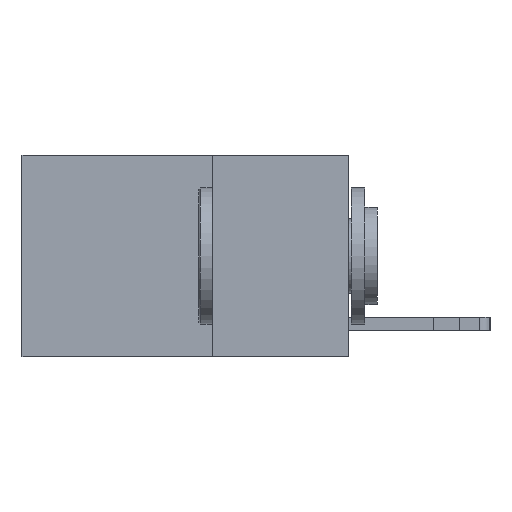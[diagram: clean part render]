
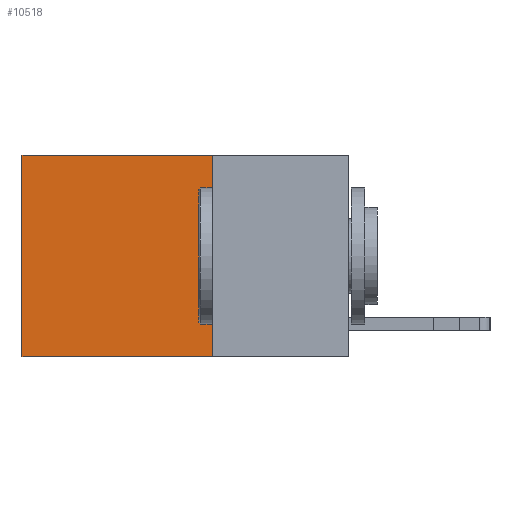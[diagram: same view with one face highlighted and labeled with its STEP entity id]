
A CAD part, left-side view. The second image highlights one B-rep face of the part: STEP entity #10518.
In plain terms, the highlighted planar face has unit normal (-1, 0, 0).
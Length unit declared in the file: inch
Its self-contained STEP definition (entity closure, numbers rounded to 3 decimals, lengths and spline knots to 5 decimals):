
#873 = ORIENTED_EDGE ( 'NONE', *, *, #3394, .F. ) ;
#1116 = VERTEX_POINT ( 'NONE', #13552 ) ;
#1158 = CARTESIAN_POINT ( 'NONE',  ( 0.2625, 0.6, 0. ) ) ;
#1653 = VECTOR ( 'NONE', #2051, 39.37008 ) ;
#2051 = DIRECTION ( 'NONE',  ( 0., 0., -1. ) ) ;
#2269 = PLANE ( 'NONE',  #6169 ) ;
#3394 = EDGE_CURVE ( 'NONE', #4470, #3804, #11139, .T. ) ;
#3656 = DIRECTION ( 'NONE',  ( 0., 1., 0. ) ) ;
#3804 = VERTEX_POINT ( 'NONE', #8317 ) ;
#4159 = ORIENTED_EDGE ( 'NONE', *, *, #14098, .F. ) ;
#4470 = VERTEX_POINT ( 'NONE', #9689 ) ;
#5174 = ORIENTED_EDGE ( 'NONE', *, *, #7414, .T. ) ;
#5525 = DIRECTION ( 'NONE',  ( 0., 0., -1. ) ) ;
#6169 = AXIS2_PLACEMENT_3D ( 'NONE', #17234, #9011, #11643 ) ;
#7014 = ORIENTED_EDGE ( 'NONE', *, *, #7881, .T. ) ;
#7414 = EDGE_CURVE ( 'NONE', #14808, #1116, #7848, .T. ) ;
#7848 = LINE ( 'NONE', #7941, #13298 ) ;
#7881 = EDGE_CURVE ( 'NONE', #1116, #3804, #11421, .T. ) ;
#7941 = CARTESIAN_POINT ( 'NONE',  ( 0.2625, 0.25, 0. ) ) ;
#8108 = EDGE_LOOP ( 'NONE', ( #7014, #873, #4159, #5174 ) ) ;
#8317 = CARTESIAN_POINT ( 'NONE',  ( 0.2625, 0.6, -0.37 ) ) ;
#9011 = DIRECTION ( 'NONE',  ( 1., 0., 0. ) ) ;
#9689 = CARTESIAN_POINT ( 'NONE',  ( 0.2625, 0.25, -0.37 ) ) ;
#9861 = CARTESIAN_POINT ( 'NONE',  ( 0.2625, 0.25, -0.37 ) ) ;
#10082 = CARTESIAN_POINT ( 'NONE',  ( 0.2625, 0.25, 0. ) ) ;
#10518 = ADVANCED_FACE ( 'NONE', ( #17154 ), #2269, .F. ) ;
#11139 = LINE ( 'NONE', #9861, #13391 ) ;
#11421 = LINE ( 'NONE', #1158, #15962 ) ;
#11643 = DIRECTION ( 'NONE',  ( 0., 0., -1. ) ) ;
#13298 = VECTOR ( 'NONE', #3656, 39.37008 ) ;
#13391 = VECTOR ( 'NONE', #14104, 39.37008 ) ;
#13552 = CARTESIAN_POINT ( 'NONE',  ( 0.2625, 0.6, 0. ) ) ;
#14098 = EDGE_CURVE ( 'NONE', #14808, #4470, #15918, .T. ) ;
#14104 = DIRECTION ( 'NONE',  ( 0., 1., 0. ) ) ;
#14377 = CARTESIAN_POINT ( 'NONE',  ( 0.2625, 0.25, 0. ) ) ;
#14808 = VERTEX_POINT ( 'NONE', #10082 ) ;
#15918 = LINE ( 'NONE', #14377, #1653 ) ;
#15962 = VECTOR ( 'NONE', #5525, 39.37008 ) ;
#17154 = FACE_OUTER_BOUND ( 'NONE', #8108, .T. ) ;
#17234 = CARTESIAN_POINT ( 'NONE',  ( 0.2625, 0.25, 0. ) ) ;
